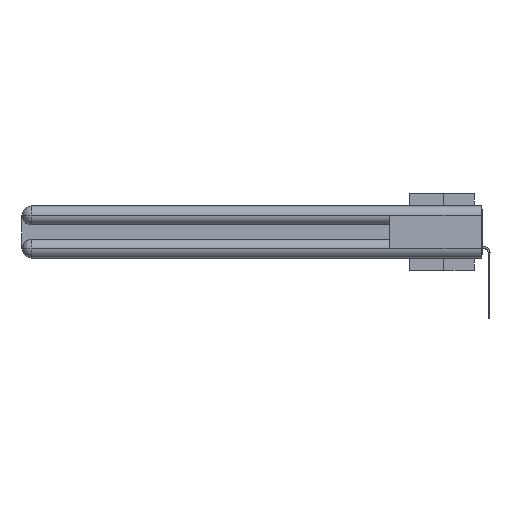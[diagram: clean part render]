
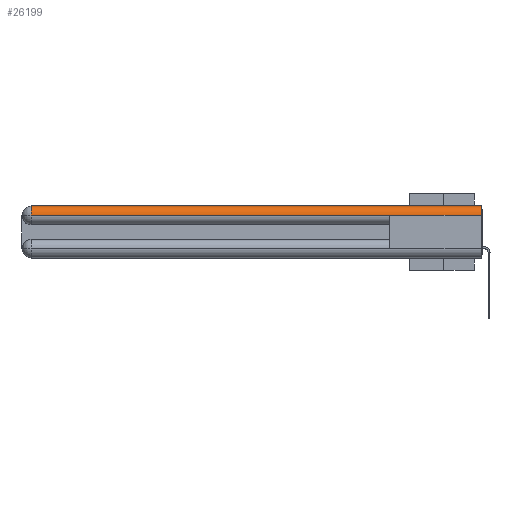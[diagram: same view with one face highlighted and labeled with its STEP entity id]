
A CAD part, left-side view. The second image highlights one B-rep face of the part: STEP entity #26199.
In plain terms, the highlighted cylindrical face has radius 1.562 mm (diameter 3.124 mm), a partial arc.
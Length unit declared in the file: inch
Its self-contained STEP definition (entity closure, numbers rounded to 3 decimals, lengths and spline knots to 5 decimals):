
#615 = AXIS2_PLACEMENT_3D ( 'NONE', #6336, #30255, #3396 ) ;
#1181 = VERTEX_POINT ( 'NONE', #24012 ) ;
#3396 = DIRECTION ( 'NONE',  ( 0., 0., 1. ) ) ;
#6336 = CARTESIAN_POINT ( 'NONE',  ( 0.0615, 0., -0.0615 ) ) ;
#8064 = EDGE_CURVE ( 'NONE', #17044, #11683, #31587, .T. ) ;
#8910 = DIRECTION ( 'NONE',  ( 0., -1., 0. ) ) ;
#9205 = CIRCLE ( 'NONE', #35399, 0.0615 ) ;
#10191 = EDGE_CURVE ( 'NONE', #11683, #1181, #32751, .T. ) ;
#11593 = DIRECTION ( 'NONE',  ( 0., 1., 0. ) ) ;
#11683 = VERTEX_POINT ( 'NONE', #22589 ) ;
#13973 = CARTESIAN_POINT ( 'NONE',  ( 0., 3., -0.0615 ) ) ;
#14222 = VECTOR ( 'NONE', #11593, 39.37008 ) ;
#15697 = CARTESIAN_POINT ( 'NONE',  ( 0., 0.6, -0.0615 ) ) ;
#16653 = VERTEX_POINT ( 'NONE', #15697 ) ;
#17044 = VERTEX_POINT ( 'NONE', #19008 ) ;
#18319 = CYLINDRICAL_SURFACE ( 'NONE', #615, 0.0615 ) ;
#19008 = CARTESIAN_POINT ( 'NONE',  ( 0.0615, 2.94, 0. ) ) ;
#19037 = AXIS2_PLACEMENT_3D ( 'NONE', #23591, #32207, #38297 ) ;
#19280 = CARTESIAN_POINT ( 'NONE',  ( 0.0615, 0., 0. ) ) ;
#19663 = DIRECTION ( 'NONE',  ( 0., -1., 0. ) ) ;
#19766 = EDGE_CURVE ( 'NONE', #26866, #16653, #37801, .T. ) ;
#20284 = EDGE_CURVE ( 'NONE', #17044, #26866, #9205, .T. ) ;
#20559 = DIRECTION ( 'NONE',  ( 0., -1., 0. ) ) ;
#21049 = VECTOR ( 'NONE', #20559, 39.37008 ) ;
#21710 = EDGE_CURVE ( 'NONE', #1181, #16653, #38451, .T. ) ;
#21903 = ORIENTED_EDGE ( 'NONE', *, *, #19766, .T. ) ;
#22589 = CARTESIAN_POINT ( 'NONE',  ( 0.0615, 0., 0. ) ) ;
#23445 = ORIENTED_EDGE ( 'NONE', *, *, #21710, .F. ) ;
#23591 = CARTESIAN_POINT ( 'NONE',  ( 0.0615, 0., -0.0615 ) ) ;
#23965 = ORIENTED_EDGE ( 'NONE', *, *, #20284, .T. ) ;
#24012 = CARTESIAN_POINT ( 'NONE',  ( 0., 0., -0.0615 ) ) ;
#26040 = CARTESIAN_POINT ( 'NONE',  ( 0., 3., -0.0615 ) ) ;
#26199 = ADVANCED_FACE ( 'NONE', ( #33177 ), #18319, .T. ) ;
#26866 = VERTEX_POINT ( 'NONE', #38205 ) ;
#28750 = ORIENTED_EDGE ( 'NONE', *, *, #10191, .F. ) ;
#30255 = DIRECTION ( 'NONE',  ( 0., 1., 0. ) ) ;
#30287 = CARTESIAN_POINT ( 'NONE',  ( 0.0615, 2.94, -0.0615 ) ) ;
#31587 = LINE ( 'NONE', #19280, #37636 ) ;
#32207 = DIRECTION ( 'NONE',  ( 0., -1., 0. ) ) ;
#32620 = DIRECTION ( 'NONE',  ( 0., 0., 1. ) ) ;
#32751 = CIRCLE ( 'NONE', #19037, 0.0615 ) ;
#33094 = ORIENTED_EDGE ( 'NONE', *, *, #8064, .F. ) ;
#33177 = FACE_OUTER_BOUND ( 'NONE', #34109, .T. ) ;
#34109 = EDGE_LOOP ( 'NONE', ( #33094, #23965, #21903, #23445, #28750 ) ) ;
#35399 = AXIS2_PLACEMENT_3D ( 'NONE', #30287, #8910, #32620 ) ;
#37636 = VECTOR ( 'NONE', #19663, 39.37008 ) ;
#37801 = LINE ( 'NONE', #26040, #21049 ) ;
#38205 = CARTESIAN_POINT ( 'NONE',  ( 0., 2.94, -0.0615 ) ) ;
#38297 = DIRECTION ( 'NONE',  ( 1., 0., 0. ) ) ;
#38451 = LINE ( 'NONE', #13973, #14222 ) ;
